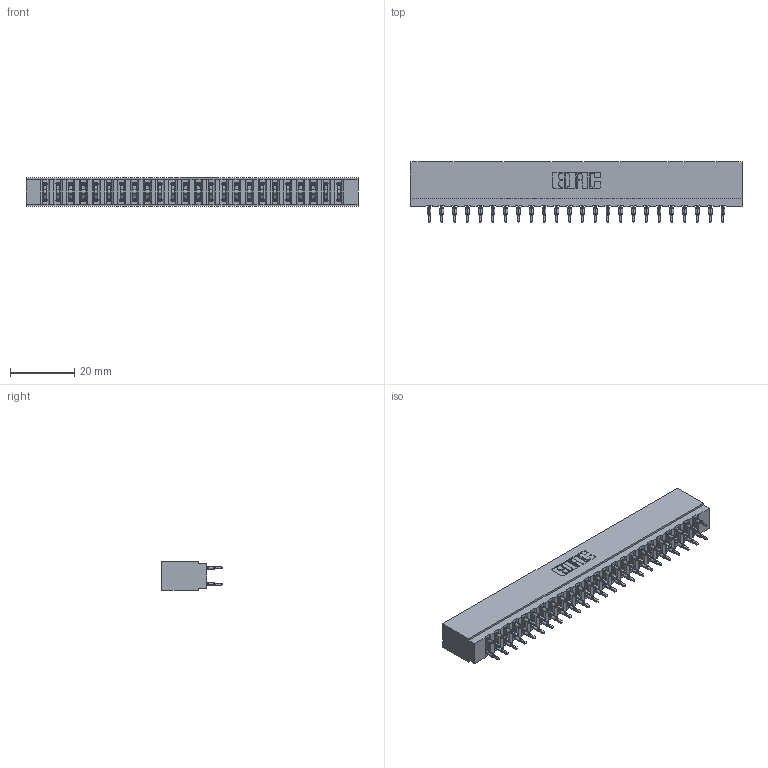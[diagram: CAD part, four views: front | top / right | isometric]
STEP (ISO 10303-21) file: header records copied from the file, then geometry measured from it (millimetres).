
FILE_DESCRIPTION (( 'STEP AP203' ), '1' );
FILE_NAME ('717-048-560-201.STEP', '2026-02-20T18:11:55', ( '' ), ( '' ), 'SwSTEP 2.0', 'SolidWorks 2023', '' );
FILE_SCHEMA (( 'CONFIG_CONTROL_DESIGN' ));
Length unit declared in the file: millimetre
Products named in the file (3): 745-292-001_560; 717-048-560-201; 717 Part_Insulator Option - 06
Assembly tree (49 placements, depth 2):
  717-048-560-201
    717 Part_Insulator Option - 06
    745-292-001_560  x48
Bounding box: 102.97 x 18.78 x 8.89 mm (x, y, z)
Volume: 9174.3 mm3; surface area: 14637.2 mm2
Topology: 49 solids, 49 shells, 4846 faces, 13259 edges, 8422 vertices
Faces by surface type: plane 2526, cylinder 1072, bspline 960, torus 288
Entity records: 43908 total; most frequent: CARTESIAN_POINT 8131, ORIENTED_EDGE 7530, DIRECTION 6595, EDGE_CURVE 3765, LINE 3431, VECTOR 3431, VERTEX_POINT 2406, AXIS2_PLACEMENT_3D 1582
